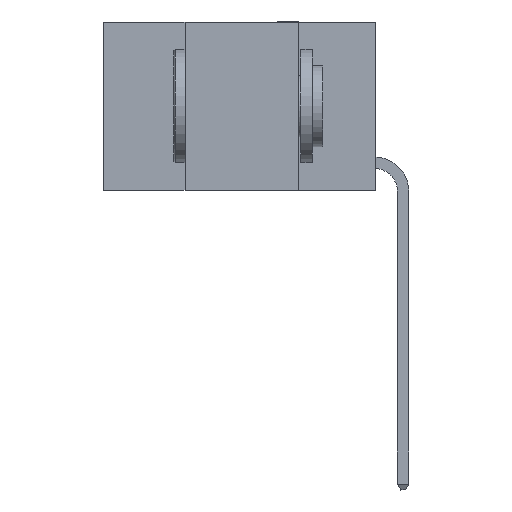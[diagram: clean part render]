
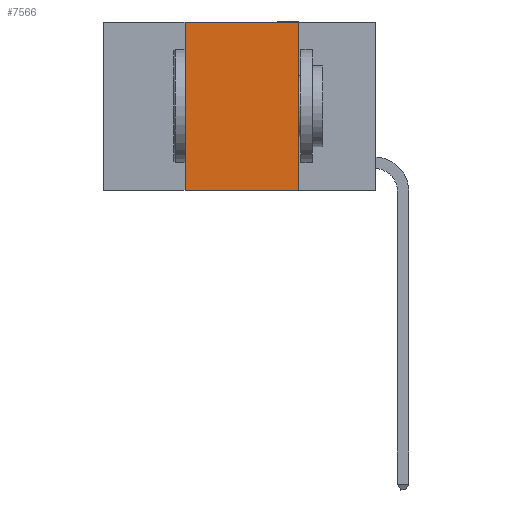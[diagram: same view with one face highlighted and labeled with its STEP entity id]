
A CAD part, left-side view. The second image highlights one B-rep face of the part: STEP entity #7566.
In plain terms, the highlighted planar face has unit normal (-1, 0, 0).
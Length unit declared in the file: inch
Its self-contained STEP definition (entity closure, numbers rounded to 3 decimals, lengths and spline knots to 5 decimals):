
#911 = CARTESIAN_POINT ( 'NONE',  ( 0., 0.42, -0.37 ) ) ;
#1146 = LINE ( 'NONE', #3983, #8256 ) ;
#1249 = DIRECTION ( 'NONE',  ( 0., -1., 0. ) ) ;
#1325 = VECTOR ( 'NONE', #11227, 39.37008 ) ;
#2462 = DIRECTION ( 'NONE',  ( 0., 0., 1. ) ) ;
#2632 = DIRECTION ( 'NONE',  ( 0., 0., -1. ) ) ;
#3051 = VECTOR ( 'NONE', #2462, 39.37008 ) ;
#3056 = CARTESIAN_POINT ( 'NONE',  ( 0., 0.17, -0.37 ) ) ;
#3210 = CARTESIAN_POINT ( 'NONE',  ( 0., 0.17, 0. ) ) ;
#3298 = LINE ( 'NONE', #4666, #7849 ) ;
#3503 = CARTESIAN_POINT ( 'NONE',  ( 0., 0.42, 0. ) ) ;
#3983 = CARTESIAN_POINT ( 'NONE',  ( 0., 0.17, 0. ) ) ;
#4529 = FACE_OUTER_BOUND ( 'NONE', #6148, .T. ) ;
#4659 = EDGE_CURVE ( 'NONE', #8978, #9026, #11332, .T. ) ;
#4666 = CARTESIAN_POINT ( 'NONE',  ( 0., 0.6, 0. ) ) ;
#5053 = ORIENTED_EDGE ( 'NONE', *, *, #4659, .F. ) ;
#5491 = VERTEX_POINT ( 'NONE', #3210 ) ;
#5494 = DIRECTION ( 'NONE',  ( 1., 0., 0. ) ) ;
#6148 = EDGE_LOOP ( 'NONE', ( #9697, #9237, #5053, #10875 ) ) ;
#6256 = CARTESIAN_POINT ( 'NONE',  ( 0., 0.6, -0.37 ) ) ;
#6548 = EDGE_CURVE ( 'NONE', #5491, #8245, #1146, .T. ) ;
#7150 = CARTESIAN_POINT ( 'NONE',  ( 0., 0.42, 0. ) ) ;
#7409 = AXIS2_PLACEMENT_3D ( 'NONE', #7482, #5494, #2632 ) ;
#7482 = CARTESIAN_POINT ( 'NONE',  ( 0., 0.6, 0. ) ) ;
#7566 = ADVANCED_FACE ( 'NONE', ( #4529 ), #9302, .F. ) ;
#7849 = VECTOR ( 'NONE', #1249, 39.37008 ) ;
#8109 = DIRECTION ( 'NONE',  ( 0., 0., -1. ) ) ;
#8245 = VERTEX_POINT ( 'NONE', #3056 ) ;
#8256 = VECTOR ( 'NONE', #8109, 39.37008 ) ;
#8303 = LINE ( 'NONE', #6256, #1325 ) ;
#8823 = EDGE_CURVE ( 'NONE', #9026, #5491, #3298, .T. ) ;
#8978 = VERTEX_POINT ( 'NONE', #911 ) ;
#9026 = VERTEX_POINT ( 'NONE', #7150 ) ;
#9237 = ORIENTED_EDGE ( 'NONE', *, *, #8823, .F. ) ;
#9302 = PLANE ( 'NONE',  #7409 ) ;
#9697 = ORIENTED_EDGE ( 'NONE', *, *, #6548, .F. ) ;
#10875 = ORIENTED_EDGE ( 'NONE', *, *, #12228, .T. ) ;
#11227 = DIRECTION ( 'NONE',  ( 0., -1., 0. ) ) ;
#11332 = LINE ( 'NONE', #3503, #3051 ) ;
#12228 = EDGE_CURVE ( 'NONE', #8978, #8245, #8303, .T. ) ;
